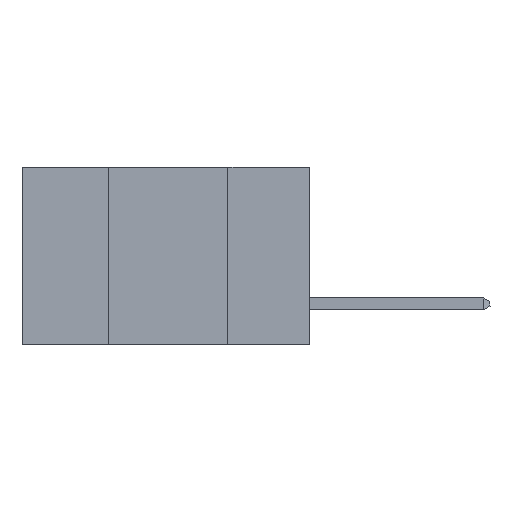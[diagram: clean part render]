
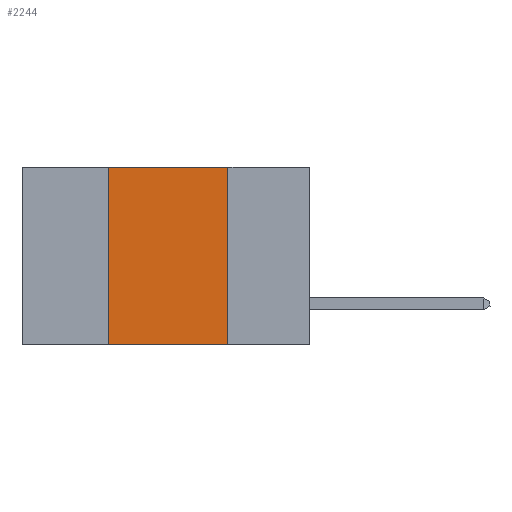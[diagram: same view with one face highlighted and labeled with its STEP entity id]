
A CAD part, left-side view. The second image highlights one B-rep face of the part: STEP entity #2244.
In plain terms, the highlighted planar face has unit normal (-1, 0, 0).
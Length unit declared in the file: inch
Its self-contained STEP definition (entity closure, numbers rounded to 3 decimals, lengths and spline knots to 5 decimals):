
#1483 = LINE ( 'NONE', #8037, #7943 ) ;
#2244 = ADVANCED_FACE ( 'NONE', ( #7950 ), #20559, .F. ) ;
#2969 = VECTOR ( 'NONE', #26757, 39.37008 ) ;
#3701 = ORIENTED_EDGE ( 'NONE', *, *, #20313, .F. ) ;
#4521 = ORIENTED_EDGE ( 'NONE', *, *, #24905, .F. ) ;
#4777 = EDGE_CURVE ( 'NONE', #22643, #24798, #1483, .T. ) ;
#5667 = DIRECTION ( 'NONE',  ( 0., 0., 1. ) ) ;
#6553 = ORIENTED_EDGE ( 'NONE', *, *, #4777, .F. ) ;
#7943 = VECTOR ( 'NONE', #5667, 39.37008 ) ;
#7950 = FACE_OUTER_BOUND ( 'NONE', #28100, .T. ) ;
#8037 = CARTESIAN_POINT ( 'NONE',  ( 0., 0.42, 0. ) ) ;
#9006 = DIRECTION ( 'NONE',  ( 1., 0., 0. ) ) ;
#11789 = VERTEX_POINT ( 'NONE', #26774 ) ;
#12094 = DIRECTION ( 'NONE',  ( 0., -1., 0. ) ) ;
#14213 = VECTOR ( 'NONE', #27330, 39.37008 ) ;
#15797 = LINE ( 'NONE', #24504, #2969 ) ;
#17115 = ORIENTED_EDGE ( 'NONE', *, *, #27708, .T. ) ;
#17548 = VERTEX_POINT ( 'NONE', #29294 ) ;
#18697 = CARTESIAN_POINT ( 'NONE',  ( 0., 0.42, -0.37 ) ) ;
#20313 = EDGE_CURVE ( 'NONE', #24798, #17548, #25732, .T. ) ;
#20559 = PLANE ( 'NONE',  #26362 ) ;
#22643 = VERTEX_POINT ( 'NONE', #18697 ) ;
#22740 = CARTESIAN_POINT ( 'NONE',  ( 0., 0.6, 0. ) ) ;
#23375 = CARTESIAN_POINT ( 'NONE',  ( 0., 0.6, 0. ) ) ;
#24211 = CARTESIAN_POINT ( 'NONE',  ( 0., 0.42, 0. ) ) ;
#24504 = CARTESIAN_POINT ( 'NONE',  ( 0., 0.17, 0. ) ) ;
#24798 = VERTEX_POINT ( 'NONE', #24211 ) ;
#24905 = EDGE_CURVE ( 'NONE', #17548, #11789, #15797, .T. ) ;
#25003 = DIRECTION ( 'NONE',  ( 0., 0., -1. ) ) ;
#25006 = VECTOR ( 'NONE', #12094, 39.37008 ) ;
#25107 = CARTESIAN_POINT ( 'NONE',  ( 0., 0.6, -0.37 ) ) ;
#25732 = LINE ( 'NONE', #23375, #25006 ) ;
#26150 = LINE ( 'NONE', #25107, #14213 ) ;
#26362 = AXIS2_PLACEMENT_3D ( 'NONE', #22740, #9006, #25003 ) ;
#26757 = DIRECTION ( 'NONE',  ( 0., 0., -1. ) ) ;
#26774 = CARTESIAN_POINT ( 'NONE',  ( 0., 0.17, -0.37 ) ) ;
#27330 = DIRECTION ( 'NONE',  ( 0., -1., 0. ) ) ;
#27708 = EDGE_CURVE ( 'NONE', #22643, #11789, #26150, .T. ) ;
#28100 = EDGE_LOOP ( 'NONE', ( #4521, #3701, #6553, #17115 ) ) ;
#29294 = CARTESIAN_POINT ( 'NONE',  ( 0., 0.17, 0. ) ) ;
